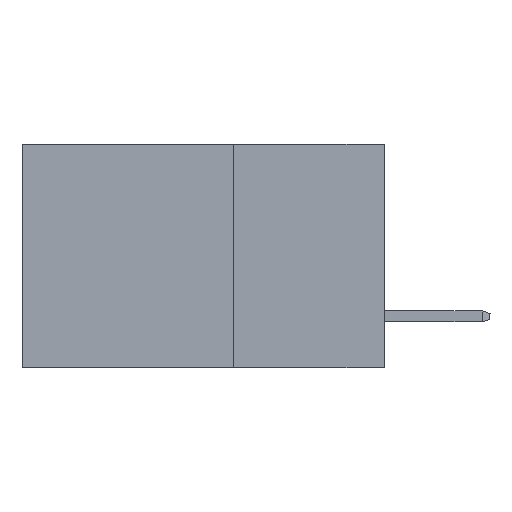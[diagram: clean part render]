
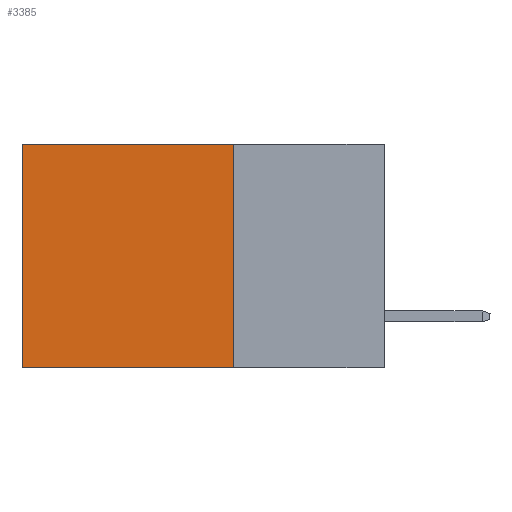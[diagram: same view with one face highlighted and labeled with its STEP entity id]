
A CAD part, left-side view. The second image highlights one B-rep face of the part: STEP entity #3385.
In plain terms, the highlighted planar face has unit normal (-1, 0, 0).
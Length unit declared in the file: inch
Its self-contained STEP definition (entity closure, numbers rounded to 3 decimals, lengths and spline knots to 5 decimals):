
#291 = VERTEX_POINT ( 'NONE', #350 ) ;
#350 = CARTESIAN_POINT ( 'NONE',  ( 0.2615, 0.6, -0.37 ) ) ;
#735 = PLANE ( 'NONE',  #1772 ) ;
#928 = VERTEX_POINT ( 'NONE', #8328 ) ;
#931 = LINE ( 'NONE', #7489, #11812 ) ;
#1092 = EDGE_CURVE ( 'NONE', #4674, #10470, #931, .T. ) ;
#1158 = CARTESIAN_POINT ( 'NONE',  ( 0.2615, 0.25, -0.37 ) ) ;
#1772 = AXIS2_PLACEMENT_3D ( 'NONE', #6103, #10766, #9040 ) ;
#1934 = LINE ( 'NONE', #4487, #9034 ) ;
#1970 = ORIENTED_EDGE ( 'NONE', *, *, #5380, .F. ) ;
#2021 = DIRECTION ( 'NONE',  ( 0., 1., 0. ) ) ;
#2130 = EDGE_CURVE ( 'NONE', #4674, #928, #8706, .T. ) ;
#2466 = DIRECTION ( 'NONE',  ( 0., 1., 0. ) ) ;
#3385 = ADVANCED_FACE ( 'NONE', ( #8031 ), #735, .F. ) ;
#4487 = CARTESIAN_POINT ( 'NONE',  ( 0.2615, 0.6, -0.37 ) ) ;
#4674 = VERTEX_POINT ( 'NONE', #9760 ) ;
#5380 = EDGE_CURVE ( 'NONE', #10470, #291, #6632, .T. ) ;
#5759 = EDGE_CURVE ( 'NONE', #928, #291, #1934, .T. ) ;
#5917 = DIRECTION ( 'NONE',  ( 0., 0., -1. ) ) ;
#6103 = CARTESIAN_POINT ( 'NONE',  ( 0.2615, 0.25, -0.37 ) ) ;
#6488 = DIRECTION ( 'NONE',  ( 0., 0., -1. ) ) ;
#6632 = LINE ( 'NONE', #1158, #10767 ) ;
#7489 = CARTESIAN_POINT ( 'NONE',  ( 0.2615, 0.25, -0.37 ) ) ;
#7500 = EDGE_LOOP ( 'NONE', ( #8878, #1970, #8715, #11393 ) ) ;
#8031 = FACE_OUTER_BOUND ( 'NONE', #7500, .T. ) ;
#8328 = CARTESIAN_POINT ( 'NONE',  ( 0.2615, 0.6, 0. ) ) ;
#8706 = LINE ( 'NONE', #9690, #11463 ) ;
#8715 = ORIENTED_EDGE ( 'NONE', *, *, #1092, .F. ) ;
#8878 = ORIENTED_EDGE ( 'NONE', *, *, #5759, .T. ) ;
#9034 = VECTOR ( 'NONE', #6488, 39.37008 ) ;
#9040 = DIRECTION ( 'NONE',  ( 0., 0., -1. ) ) ;
#9690 = CARTESIAN_POINT ( 'NONE',  ( 0.2615, 0.25, 0. ) ) ;
#9760 = CARTESIAN_POINT ( 'NONE',  ( 0.2615, 0.25, 0. ) ) ;
#10470 = VERTEX_POINT ( 'NONE', #11772 ) ;
#10766 = DIRECTION ( 'NONE',  ( 1., 0., 0. ) ) ;
#10767 = VECTOR ( 'NONE', #2021, 39.37008 ) ;
#11393 = ORIENTED_EDGE ( 'NONE', *, *, #2130, .T. ) ;
#11463 = VECTOR ( 'NONE', #2466, 39.37008 ) ;
#11772 = CARTESIAN_POINT ( 'NONE',  ( 0.2615, 0.25, -0.37 ) ) ;
#11812 = VECTOR ( 'NONE', #5917, 39.37008 ) ;
